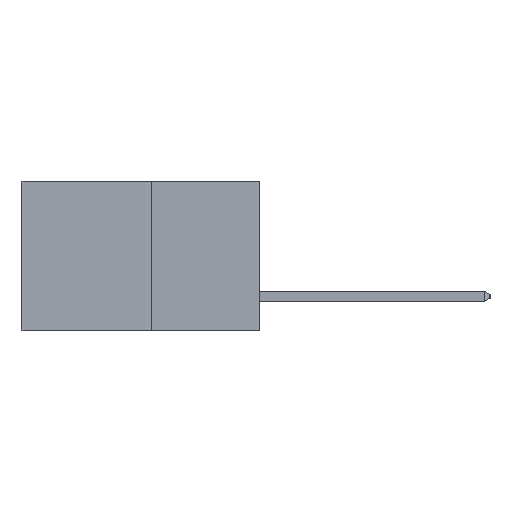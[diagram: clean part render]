
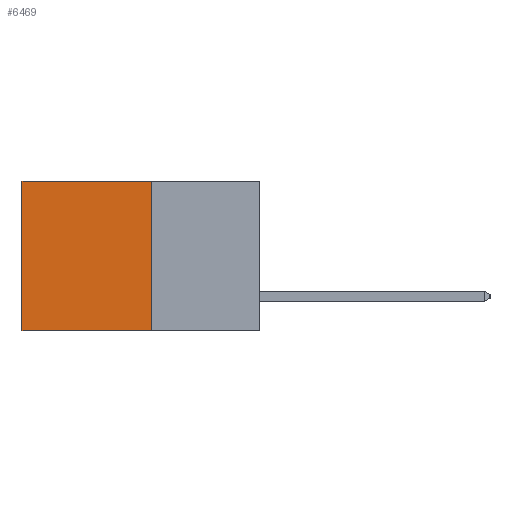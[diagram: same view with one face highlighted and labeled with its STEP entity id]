
A CAD part, left-side view. The second image highlights one B-rep face of the part: STEP entity #6469.
In plain terms, the highlighted planar face has unit normal (-1, 0, 0).
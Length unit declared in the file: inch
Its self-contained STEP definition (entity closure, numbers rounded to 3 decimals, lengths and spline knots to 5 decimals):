
#2103 = DIRECTION ( 'NONE',  ( 0., 0., -1. ) ) ;
#2119 = CARTESIAN_POINT ( 'NONE',  ( 0.277, 0.27, -0.37 ) ) ;
#2411 = CARTESIAN_POINT ( 'NONE',  ( 0.277, 0.27, -0.37 ) ) ;
#2613 = EDGE_CURVE ( 'NONE', #10503, #15246, #6827, .T. ) ;
#3394 = VECTOR ( 'NONE', #5958, 39.37008 ) ;
#3433 = DIRECTION ( 'NONE',  ( 0., 1., 0. ) ) ;
#4770 = CARTESIAN_POINT ( 'NONE',  ( 0.277, 0.59, -0.37 ) ) ;
#5370 = EDGE_CURVE ( 'NONE', #7722, #5534, #12446, .T. ) ;
#5380 = ORIENTED_EDGE ( 'NONE', *, *, #6945, .F. ) ;
#5534 = VERTEX_POINT ( 'NONE', #16445 ) ;
#5604 = VECTOR ( 'NONE', #3433, 39.37008 ) ;
#5765 = ORIENTED_EDGE ( 'NONE', *, *, #5370, .T. ) ;
#5958 = DIRECTION ( 'NONE',  ( 0., 1., 0. ) ) ;
#6251 = VECTOR ( 'NONE', #15704, 39.37008 ) ;
#6350 = AXIS2_PLACEMENT_3D ( 'NONE', #12901, #12629, #12626 ) ;
#6469 = ADVANCED_FACE ( 'NONE', ( #9622 ), #12923, .F. ) ;
#6827 = LINE ( 'NONE', #12542, #3394 ) ;
#6945 = EDGE_CURVE ( 'NONE', #7722, #10503, #12980, .T. ) ;
#7603 = ORIENTED_EDGE ( 'NONE', *, *, #2613, .F. ) ;
#7722 = VERTEX_POINT ( 'NONE', #11588 ) ;
#9622 = FACE_OUTER_BOUND ( 'NONE', #10434, .T. ) ;
#10190 = ORIENTED_EDGE ( 'NONE', *, *, #10242, .T. ) ;
#10242 = EDGE_CURVE ( 'NONE', #5534, #15246, #16308, .T. ) ;
#10434 = EDGE_LOOP ( 'NONE', ( #10190, #7603, #5380, #5765 ) ) ;
#10503 = VERTEX_POINT ( 'NONE', #2119 ) ;
#11140 = CARTESIAN_POINT ( 'NONE',  ( 0.277, 0.27, 0. ) ) ;
#11588 = CARTESIAN_POINT ( 'NONE',  ( 0.277, 0.27, 0. ) ) ;
#12446 = LINE ( 'NONE', #11140, #5604 ) ;
#12542 = CARTESIAN_POINT ( 'NONE',  ( 0.277, 0.27, -0.37 ) ) ;
#12626 = DIRECTION ( 'NONE',  ( 0., 0., -1. ) ) ;
#12629 = DIRECTION ( 'NONE',  ( 1., 0., 0. ) ) ;
#12901 = CARTESIAN_POINT ( 'NONE',  ( 0.277, 0.27, -0.37 ) ) ;
#12923 = PLANE ( 'NONE',  #6350 ) ;
#12980 = LINE ( 'NONE', #2411, #16211 ) ;
#14498 = CARTESIAN_POINT ( 'NONE',  ( 0.277, 0.59, -0.37 ) ) ;
#15246 = VERTEX_POINT ( 'NONE', #4770 ) ;
#15704 = DIRECTION ( 'NONE',  ( 0., 0., -1. ) ) ;
#16211 = VECTOR ( 'NONE', #2103, 39.37008 ) ;
#16308 = LINE ( 'NONE', #14498, #6251 ) ;
#16445 = CARTESIAN_POINT ( 'NONE',  ( 0.277, 0.59, 0. ) ) ;
